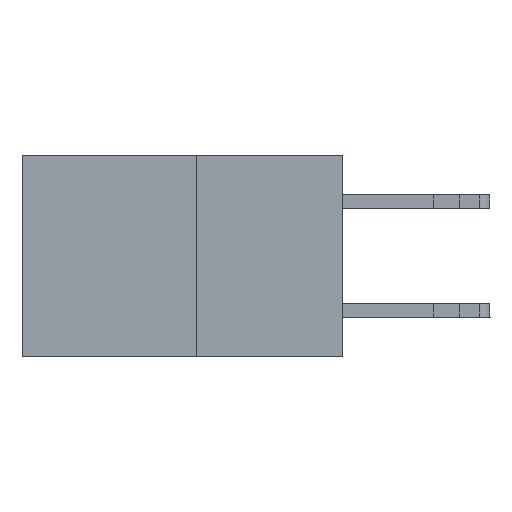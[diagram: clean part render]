
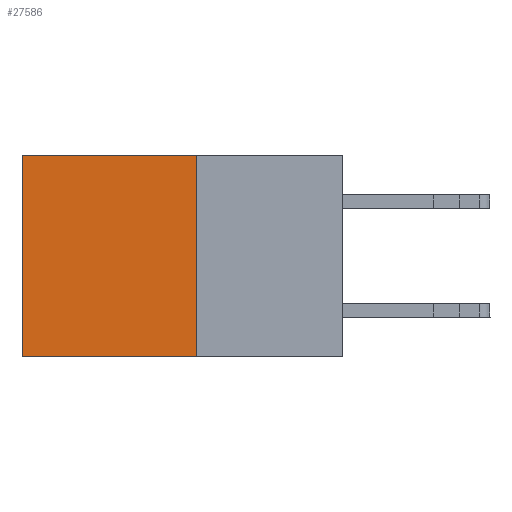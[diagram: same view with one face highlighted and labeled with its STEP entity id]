
A CAD part, left-side view. The second image highlights one B-rep face of the part: STEP entity #27586.
In plain terms, the highlighted planar face has unit normal (-1, 0, 0).
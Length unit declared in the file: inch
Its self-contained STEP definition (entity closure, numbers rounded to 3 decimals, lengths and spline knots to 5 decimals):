
#3775 = VERTEX_POINT ( 'NONE', #6395 ) ;
#4081 = DIRECTION ( 'NONE',  ( 0., 0., -1. ) ) ;
#5281 = CARTESIAN_POINT ( 'NONE',  ( 0.277, 0.27, 0. ) ) ;
#5768 = ORIENTED_EDGE ( 'NONE', *, *, #31627, .T. ) ;
#6087 = CARTESIAN_POINT ( 'NONE',  ( 0.277, 0.59, 0. ) ) ;
#6395 = CARTESIAN_POINT ( 'NONE',  ( 0.277, 0.59, -0.37 ) ) ;
#7191 = CARTESIAN_POINT ( 'NONE',  ( 0.277, 0.27, -0.37 ) ) ;
#9263 = DIRECTION ( 'NONE',  ( 0., 0., -1. ) ) ;
#9474 = VECTOR ( 'NONE', #4081, 39.37008 ) ;
#9879 = DIRECTION ( 'NONE',  ( 0., 0., -1. ) ) ;
#9986 = ORIENTED_EDGE ( 'NONE', *, *, #25009, .F. ) ;
#12207 = CARTESIAN_POINT ( 'NONE',  ( 0.277, 0.27, 0. ) ) ;
#13831 = FACE_OUTER_BOUND ( 'NONE', #23959, .T. ) ;
#13836 = LINE ( 'NONE', #5281, #19190 ) ;
#15811 = CARTESIAN_POINT ( 'NONE',  ( 0.277, 0.27, -0.37 ) ) ;
#17322 = LINE ( 'NONE', #22585, #9474 ) ;
#17714 = PLANE ( 'NONE',  #31629 ) ;
#18055 = VECTOR ( 'NONE', #31623, 39.37008 ) ;
#18575 = DIRECTION ( 'NONE',  ( 0., 1., 0. ) ) ;
#18609 = VERTEX_POINT ( 'NONE', #12207 ) ;
#19190 = VECTOR ( 'NONE', #18575, 39.37008 ) ;
#20262 = VERTEX_POINT ( 'NONE', #33959 ) ;
#20576 = EDGE_CURVE ( 'NONE', #22730, #3775, #17322, .T. ) ;
#22438 = CARTESIAN_POINT ( 'NONE',  ( 0.277, 0.27, -0.37 ) ) ;
#22585 = CARTESIAN_POINT ( 'NONE',  ( 0.277, 0.59, -0.37 ) ) ;
#22730 = VERTEX_POINT ( 'NONE', #6087 ) ;
#23324 = ORIENTED_EDGE ( 'NONE', *, *, #20576, .T. ) ;
#23959 = EDGE_LOOP ( 'NONE', ( #23324, #9986, #31830, #5768 ) ) ;
#25009 = EDGE_CURVE ( 'NONE', #20262, #3775, #32909, .T. ) ;
#25632 = VECTOR ( 'NONE', #9263, 39.37008 ) ;
#25686 = DIRECTION ( 'NONE',  ( 1., 0., 0. ) ) ;
#27586 = ADVANCED_FACE ( 'NONE', ( #13831 ), #17714, .F. ) ;
#29646 = EDGE_CURVE ( 'NONE', #18609, #20262, #31825, .T. ) ;
#31623 = DIRECTION ( 'NONE',  ( 0., 1., 0. ) ) ;
#31627 = EDGE_CURVE ( 'NONE', #18609, #22730, #13836, .T. ) ;
#31629 = AXIS2_PLACEMENT_3D ( 'NONE', #7191, #25686, #9879 ) ;
#31825 = LINE ( 'NONE', #22438, #25632 ) ;
#31830 = ORIENTED_EDGE ( 'NONE', *, *, #29646, .F. ) ;
#32909 = LINE ( 'NONE', #15811, #18055 ) ;
#33959 = CARTESIAN_POINT ( 'NONE',  ( 0.277, 0.27, -0.37 ) ) ;
